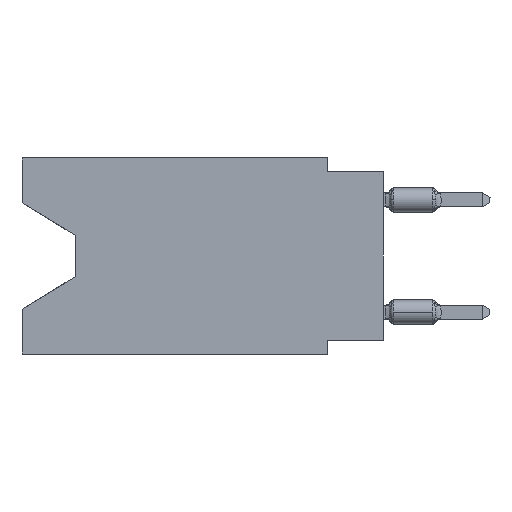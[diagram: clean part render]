
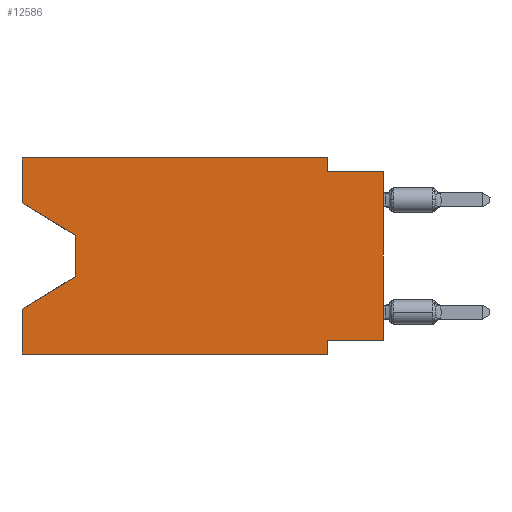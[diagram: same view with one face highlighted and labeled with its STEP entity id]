
A CAD part, left-side view. The second image highlights one B-rep face of the part: STEP entity #12586.
In plain terms, the highlighted planar face has unit normal (-1, 0, 0).
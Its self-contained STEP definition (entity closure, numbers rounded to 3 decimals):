
#219 = DIRECTION ( 'NONE',  ( 0., -1., 0. ) ) ;
#352 = VERTEX_POINT ( 'NONE', #23289 ) ;
#457 = FACE_OUTER_BOUND ( 'NONE', #22246, .T. ) ;
#1435 = DIRECTION ( 'NONE',  ( 0., 0., -1. ) ) ;
#1455 = ORIENTED_EDGE ( 'NONE', *, *, #28264, .T. ) ;
#1757 = CARTESIAN_POINT ( 'NONE',  ( 0., 16.383, -8.89 ) ) ;
#2263 = CARTESIAN_POINT ( 'NONE',  ( 0., 16.383, -2.038 ) ) ;
#2398 = DIRECTION ( 'NONE',  ( 0., -0.855, -0.519 ) ) ;
#2441 = EDGE_CURVE ( 'NONE', #19419, #11750, #26460, .T. ) ;
#2753 = VERTEX_POINT ( 'NONE', #23040 ) ;
#4181 = ORIENTED_EDGE ( 'NONE', *, *, #16460, .T. ) ;
#4607 = EDGE_CURVE ( 'NONE', #18739, #14104, #28730, .T. ) ;
#4671 = ORIENTED_EDGE ( 'NONE', *, *, #4607, .F. ) ;
#4762 = CARTESIAN_POINT ( 'NONE',  ( 0., 13.97, -5.385 ) ) ;
#6487 = EDGE_CURVE ( 'NONE', #2753, #17919, #14193, .T. ) ;
#6530 = CARTESIAN_POINT ( 'NONE',  ( 0., 0., -8.255 ) ) ;
#6587 = LINE ( 'NONE', #8502, #19555 ) ;
#7567 = VECTOR ( 'NONE', #8652, 1000. ) ;
#7585 = CARTESIAN_POINT ( 'NONE',  ( 0., 2.54, -8.89 ) ) ;
#7841 = CARTESIAN_POINT ( 'NONE',  ( 0., 16.383, -2.038 ) ) ;
#8397 = VERTEX_POINT ( 'NONE', #21927 ) ;
#8424 = EDGE_CURVE ( 'NONE', #19419, #8397, #13561, .T. ) ;
#8477 = EDGE_CURVE ( 'NONE', #352, #2753, #26620, .T. ) ;
#8502 = CARTESIAN_POINT ( 'NONE',  ( 0., 13.97, -5.385 ) ) ;
#8571 = DIRECTION ( 'NONE',  ( 0., -1., 0. ) ) ;
#8652 = DIRECTION ( 'NONE',  ( 0., 0., -1. ) ) ;
#9705 = DIRECTION ( 'NONE',  ( 1., 0., 0. ) ) ;
#9865 = EDGE_CURVE ( 'NONE', #8397, #15323, #28872, .T. ) ;
#10402 = CARTESIAN_POINT ( 'NONE',  ( 0., 16.383, 0. ) ) ;
#10776 = DIRECTION ( 'NONE',  ( 0., 0., 1. ) ) ;
#10940 = CARTESIAN_POINT ( 'NONE',  ( 0., 2.54, -8.89 ) ) ;
#11069 = VERTEX_POINT ( 'NONE', #1757 ) ;
#11593 = CARTESIAN_POINT ( 'NONE',  ( 0., 16.383, 0. ) ) ;
#11750 = VERTEX_POINT ( 'NONE', #12377 ) ;
#12310 = VECTOR ( 'NONE', #25597, 1000. ) ;
#12377 = CARTESIAN_POINT ( 'NONE',  ( 0., 16.383, 0. ) ) ;
#12586 = ADVANCED_FACE ( 'NONE', ( #457 ), #28123, .F. ) ;
#12602 = ORIENTED_EDGE ( 'NONE', *, *, #6487, .F. ) ;
#12911 = VECTOR ( 'NONE', #15763, 1000. ) ;
#13561 = LINE ( 'NONE', #2263, #13850 ) ;
#13573 = LINE ( 'NONE', #16367, #24650 ) ;
#13850 = VECTOR ( 'NONE', #2398, 1000. ) ;
#14104 = VERTEX_POINT ( 'NONE', #22504 ) ;
#14193 = LINE ( 'NONE', #7585, #18195 ) ;
#14656 = DIRECTION ( 'NONE',  ( 0., 0., 1. ) ) ;
#15323 = VERTEX_POINT ( 'NONE', #4762 ) ;
#15380 = VECTOR ( 'NONE', #28144, 1000. ) ;
#15531 = CARTESIAN_POINT ( 'NONE',  ( 0., 13.97, -3.505 ) ) ;
#15763 = DIRECTION ( 'NONE',  ( 0., 1., 0. ) ) ;
#16015 = CARTESIAN_POINT ( 'NONE',  ( 0., 16.383, -6.852 ) ) ;
#16291 = ORIENTED_EDGE ( 'NONE', *, *, #8424, .T. ) ;
#16367 = CARTESIAN_POINT ( 'NONE',  ( 0., 16.383, -8.89 ) ) ;
#16460 = EDGE_CURVE ( 'NONE', #15323, #21368, #6587, .T. ) ;
#17714 = CARTESIAN_POINT ( 'NONE',  ( 0., 0., -0.635 ) ) ;
#17919 = VERTEX_POINT ( 'NONE', #10940 ) ;
#18178 = VECTOR ( 'NONE', #14656, 1000. ) ;
#18195 = VECTOR ( 'NONE', #25047, 1000. ) ;
#18545 = EDGE_CURVE ( 'NONE', #352, #20365, #21993, .T. ) ;
#18618 = EDGE_CURVE ( 'NONE', #11069, #21368, #21688, .T. ) ;
#18739 = VERTEX_POINT ( 'NONE', #22693 ) ;
#18854 = LINE ( 'NONE', #27790, #12310 ) ;
#19214 = CARTESIAN_POINT ( 'NONE',  ( 0., 0., 0. ) ) ;
#19419 = VERTEX_POINT ( 'NONE', #7841 ) ;
#19555 = VECTOR ( 'NONE', #28877, 1000. ) ;
#19859 = LINE ( 'NONE', #28801, #28245 ) ;
#20365 = VERTEX_POINT ( 'NONE', #17714 ) ;
#20863 = EDGE_CURVE ( 'NONE', #11750, #18739, #19859, .T. ) ;
#21368 = VERTEX_POINT ( 'NONE', #16015 ) ;
#21688 = LINE ( 'NONE', #10402, #18178 ) ;
#21927 = CARTESIAN_POINT ( 'NONE',  ( 0., 13.97, -3.505 ) ) ;
#21993 = LINE ( 'NONE', #19214, #15380 ) ;
#22246 = EDGE_LOOP ( 'NONE', ( #16291, #23426, #4181, #22442, #1455, #12602, #28651, #22263, #27982, #4671, #26891, #26943 ) ) ;
#22263 = ORIENTED_EDGE ( 'NONE', *, *, #18545, .T. ) ;
#22421 = EDGE_CURVE ( 'NONE', #14104, #20365, #18854, .T. ) ;
#22442 = ORIENTED_EDGE ( 'NONE', *, *, #18618, .F. ) ;
#22504 = CARTESIAN_POINT ( 'NONE',  ( 0., 2.54, -0.635 ) ) ;
#22693 = CARTESIAN_POINT ( 'NONE',  ( 0., 2.54, 0. ) ) ;
#23040 = CARTESIAN_POINT ( 'NONE',  ( 0., 2.54, -8.255 ) ) ;
#23289 = CARTESIAN_POINT ( 'NONE',  ( 0., 0., -8.255 ) ) ;
#23304 = AXIS2_PLACEMENT_3D ( 'NONE', #11593, #9705, #1435 ) ;
#23426 = ORIENTED_EDGE ( 'NONE', *, *, #9865, .T. ) ;
#23963 = CARTESIAN_POINT ( 'NONE',  ( 0., 16.383, 0. ) ) ;
#24196 = DIRECTION ( 'NONE',  ( 0., 0., -1. ) ) ;
#24650 = VECTOR ( 'NONE', #219, 1000. ) ;
#25047 = DIRECTION ( 'NONE',  ( 0., 0., -1. ) ) ;
#25597 = DIRECTION ( 'NONE',  ( 0., -1., 0. ) ) ;
#26460 = LINE ( 'NONE', #23963, #28778 ) ;
#26556 = VECTOR ( 'NONE', #24196, 1000. ) ;
#26620 = LINE ( 'NONE', #6530, #12911 ) ;
#26891 = ORIENTED_EDGE ( 'NONE', *, *, #20863, .F. ) ;
#26943 = ORIENTED_EDGE ( 'NONE', *, *, #2441, .F. ) ;
#27790 = CARTESIAN_POINT ( 'NONE',  ( 0., 0., -0.635 ) ) ;
#27982 = ORIENTED_EDGE ( 'NONE', *, *, #22421, .F. ) ;
#28123 = PLANE ( 'NONE',  #23304 ) ;
#28144 = DIRECTION ( 'NONE',  ( 0., 0., 1. ) ) ;
#28245 = VECTOR ( 'NONE', #8571, 1000. ) ;
#28264 = EDGE_CURVE ( 'NONE', #11069, #17919, #13573, .T. ) ;
#28297 = CARTESIAN_POINT ( 'NONE',  ( 0., 2.54, 0. ) ) ;
#28651 = ORIENTED_EDGE ( 'NONE', *, *, #8477, .F. ) ;
#28730 = LINE ( 'NONE', #28297, #7567 ) ;
#28778 = VECTOR ( 'NONE', #10776, 1000. ) ;
#28801 = CARTESIAN_POINT ( 'NONE',  ( 0., 16.383, 0. ) ) ;
#28872 = LINE ( 'NONE', #15531, #26556 ) ;
#28877 = DIRECTION ( 'NONE',  ( 0., 0.855, -0.519 ) ) ;
